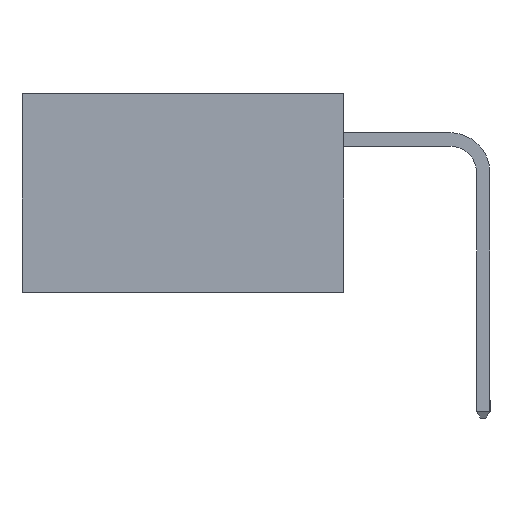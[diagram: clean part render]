
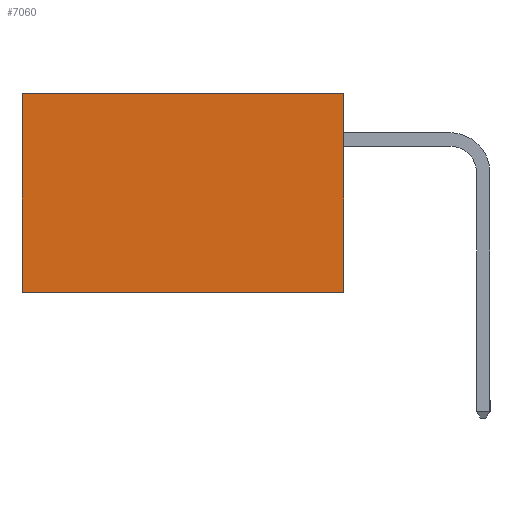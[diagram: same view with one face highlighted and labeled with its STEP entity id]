
A CAD part, left-side view. The second image highlights one B-rep face of the part: STEP entity #7060.
In plain terms, the highlighted planar face has unit normal (-1, 0, 0).
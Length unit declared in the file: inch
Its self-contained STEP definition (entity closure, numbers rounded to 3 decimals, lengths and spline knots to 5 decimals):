
#176 = VECTOR ( 'NONE', #5061, 39.37008 ) ;
#267 = ORIENTED_EDGE ( 'NONE', *, *, #17850, .F. ) ;
#609 = CARTESIAN_POINT ( 'NONE',  ( 0.2615, 0., 0. ) ) ;
#641 = DIRECTION ( 'NONE',  ( 0., 0., -1. ) ) ;
#669 = DIRECTION ( 'NONE',  ( 1., 0., 0. ) ) ;
#740 = DIRECTION ( 'NONE',  ( 0., 1., 0. ) ) ;
#1021 = PLANE ( 'NONE',  #11266 ) ;
#1670 = DIRECTION ( 'NONE',  ( 0., 0., -1. ) ) ;
#1682 = CARTESIAN_POINT ( 'NONE',  ( 0.2615, 0.6, -0.37 ) ) ;
#1974 = VERTEX_POINT ( 'NONE', #17817 ) ;
#2626 = CARTESIAN_POINT ( 'NONE',  ( 0.2615, 0., -0.37 ) ) ;
#3412 = VECTOR ( 'NONE', #1670, 39.37008 ) ;
#4202 = LINE ( 'NONE', #12306, #176 ) ;
#4856 = VERTEX_POINT ( 'NONE', #15121 ) ;
#4909 = CARTESIAN_POINT ( 'NONE',  ( 0.2615, 0., -0.37 ) ) ;
#5061 = DIRECTION ( 'NONE',  ( 0., 1., 0. ) ) ;
#5598 = CARTESIAN_POINT ( 'NONE',  ( 0.2615, 0.6, -0.37 ) ) ;
#5846 = VECTOR ( 'NONE', #740, 39.37008 ) ;
#6395 = DIRECTION ( 'NONE',  ( 0., 0., -1. ) ) ;
#7002 = EDGE_LOOP ( 'NONE', ( #11253, #18278, #267, #8818 ) ) ;
#7043 = EDGE_CURVE ( 'NONE', #4856, #16284, #18648, .T. ) ;
#7060 = ADVANCED_FACE ( 'NONE', ( #18229 ), #1021, .F. ) ;
#7928 = VERTEX_POINT ( 'NONE', #14547 ) ;
#8818 = ORIENTED_EDGE ( 'NONE', *, *, #9541, .T. ) ;
#9541 = EDGE_CURVE ( 'NONE', #7928, #4856, #9750, .T. ) ;
#9750 = LINE ( 'NONE', #609, #5846 ) ;
#10691 = VECTOR ( 'NONE', #6395, 39.37008 ) ;
#11253 = ORIENTED_EDGE ( 'NONE', *, *, #7043, .T. ) ;
#11266 = AXIS2_PLACEMENT_3D ( 'NONE', #2626, #669, #641 ) ;
#12306 = CARTESIAN_POINT ( 'NONE',  ( 0.2615, 0., -0.37 ) ) ;
#13394 = EDGE_CURVE ( 'NONE', #1974, #16284, #4202, .T. ) ;
#14547 = CARTESIAN_POINT ( 'NONE',  ( 0.2615, 0., 0. ) ) ;
#15121 = CARTESIAN_POINT ( 'NONE',  ( 0.2615, 0.6, 0. ) ) ;
#16284 = VERTEX_POINT ( 'NONE', #5598 ) ;
#17817 = CARTESIAN_POINT ( 'NONE',  ( 0.2615, 0., -0.37 ) ) ;
#17850 = EDGE_CURVE ( 'NONE', #7928, #1974, #18128, .T. ) ;
#18128 = LINE ( 'NONE', #4909, #10691 ) ;
#18229 = FACE_OUTER_BOUND ( 'NONE', #7002, .T. ) ;
#18278 = ORIENTED_EDGE ( 'NONE', *, *, #13394, .F. ) ;
#18648 = LINE ( 'NONE', #1682, #3412 ) ;
